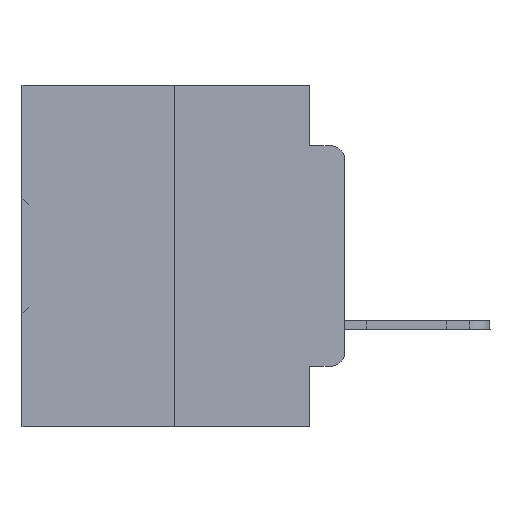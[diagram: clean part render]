
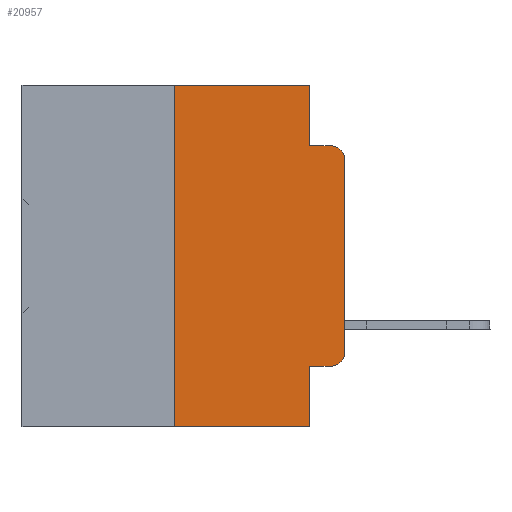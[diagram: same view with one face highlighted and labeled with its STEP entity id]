
A CAD part, left-side view. The second image highlights one B-rep face of the part: STEP entity #20957.
In plain terms, the highlighted planar face has unit normal (-1, 0, 0).
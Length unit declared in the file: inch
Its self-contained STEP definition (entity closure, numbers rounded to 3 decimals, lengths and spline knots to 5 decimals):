
#262 = DIRECTION ( 'NONE',  ( 0., -1., 0. ) ) ;
#642 = EDGE_CURVE ( 'NONE', #31950, #31048, #36042, .T. ) ;
#1874 = DIRECTION ( 'NONE',  ( -1., 0., 0. ) ) ;
#1980 = EDGE_CURVE ( 'NONE', #3647, #34408, #6090, .T. ) ;
#2743 = ORIENTED_EDGE ( 'NONE', *, *, #1980, .F. ) ;
#2965 = ORIENTED_EDGE ( 'NONE', *, *, #6004, .T. ) ;
#3647 = VERTEX_POINT ( 'NONE', #27673 ) ;
#4085 = VECTOR ( 'NONE', #11490, 39.37008 ) ;
#4771 = EDGE_CURVE ( 'NONE', #16785, #33206, #8802, .T. ) ;
#5442 = ORIENTED_EDGE ( 'NONE', *, *, #27793, .F. ) ;
#6004 = EDGE_CURVE ( 'NONE', #22142, #33494, #24230, .T. ) ;
#6090 = LINE ( 'NONE', #29186, #32910 ) ;
#6356 = PLANE ( 'NONE',  #19938 ) ;
#7488 = EDGE_LOOP ( 'NONE', ( #9934, #19368, #13056, #5442, #2743, #19041, #13561, #19748, #2965, #9713 ) ) ;
#7944 = CIRCLE ( 'NONE', #23440, 0.02 ) ;
#8224 = VECTOR ( 'NONE', #30448, 39.37008 ) ;
#8802 = LINE ( 'NONE', #28717, #4085 ) ;
#8894 = DIRECTION ( 'NONE',  ( 0., -1., 0. ) ) ;
#9002 = LINE ( 'NONE', #22781, #23582 ) ;
#9028 = DIRECTION ( 'NONE',  ( -1., 0., 0. ) ) ;
#9069 = VERTEX_POINT ( 'NONE', #16126 ) ;
#9713 = ORIENTED_EDGE ( 'NONE', *, *, #20241, .T. ) ;
#9934 = ORIENTED_EDGE ( 'NONE', *, *, #642, .T. ) ;
#10415 = VERTEX_POINT ( 'NONE', #25073 ) ;
#10775 = EDGE_CURVE ( 'NONE', #16785, #3647, #13095, .T. ) ;
#10931 = CARTESIAN_POINT ( 'NONE',  ( 0., 0.02, -0.4115 ) ) ;
#11490 = DIRECTION ( 'NONE',  ( 0., -1., 0. ) ) ;
#13056 = ORIENTED_EDGE ( 'NONE', *, *, #24681, .F. ) ;
#13095 = LINE ( 'NONE', #13651, #34116 ) ;
#13189 = DIRECTION ( 'NONE',  ( 0., 0., -1. ) ) ;
#13380 = CARTESIAN_POINT ( 'NONE',  ( 0., 0.051, -0.4115 ) ) ;
#13561 = ORIENTED_EDGE ( 'NONE', *, *, #4771, .T. ) ;
#13651 = CARTESIAN_POINT ( 'NONE',  ( 0., 0.25, 0. ) ) ;
#14601 = CARTESIAN_POINT ( 'NONE',  ( 0., 0.02, -0.1085 ) ) ;
#14711 = DIRECTION ( 'NONE',  ( 1., 0., 0. ) ) ;
#15269 = FACE_OUTER_BOUND ( 'NONE', #7488, .T. ) ;
#16126 = CARTESIAN_POINT ( 'NONE',  ( 0., 0.051, -0.0885 ) ) ;
#16474 = DIRECTION ( 'NONE',  ( 0., 0., 1. ) ) ;
#16520 = AXIS2_PLACEMENT_3D ( 'NONE', #14601, #9028, #20409 ) ;
#16656 = CARTESIAN_POINT ( 'NONE',  ( 0., 0.25, -0.5 ) ) ;
#16785 = VERTEX_POINT ( 'NONE', #16656 ) ;
#19041 = ORIENTED_EDGE ( 'NONE', *, *, #10775, .F. ) ;
#19187 = DIRECTION ( 'NONE',  ( 0., -1., 0. ) ) ;
#19368 = ORIENTED_EDGE ( 'NONE', *, *, #29441, .T. ) ;
#19748 = ORIENTED_EDGE ( 'NONE', *, *, #23740, .F. ) ;
#19938 = AXIS2_PLACEMENT_3D ( 'NONE', #20718, #14711, #26094 ) ;
#20034 = LINE ( 'NONE', #28582, #25477 ) ;
#20241 = EDGE_CURVE ( 'NONE', #33494, #31950, #7944, .T. ) ;
#20409 = DIRECTION ( 'NONE',  ( 0., 0., -1. ) ) ;
#20718 = CARTESIAN_POINT ( 'NONE',  ( 0., 0.473, 0. ) ) ;
#20864 = DIRECTION ( 'NONE',  ( 0., 0., -1. ) ) ;
#20957 = ADVANCED_FACE ( 'NONE', ( #15269 ), #6356, .F. ) ;
#21107 = CARTESIAN_POINT ( 'NONE',  ( 0., 0., -0.1085 ) ) ;
#22142 = VERTEX_POINT ( 'NONE', #27848 ) ;
#22545 = CARTESIAN_POINT ( 'NONE',  ( 0., 0.051, -0.5 ) ) ;
#22781 = CARTESIAN_POINT ( 'NONE',  ( 0., 0.051, 0. ) ) ;
#23440 = AXIS2_PLACEMENT_3D ( 'NONE', #27391, #1874, #13189 ) ;
#23582 = VECTOR ( 'NONE', #26139, 39.37008 ) ;
#23740 = EDGE_CURVE ( 'NONE', #22142, #33206, #31070, .T. ) ;
#24230 = LINE ( 'NONE', #13380, #30600 ) ;
#24681 = EDGE_CURVE ( 'NONE', #9069, #10415, #20034, .T. ) ;
#25073 = CARTESIAN_POINT ( 'NONE',  ( 0., 0.02, -0.0885 ) ) ;
#25477 = VECTOR ( 'NONE', #262, 39.37008 ) ;
#26094 = DIRECTION ( 'NONE',  ( 0., 0., -1. ) ) ;
#26139 = DIRECTION ( 'NONE',  ( 0., 0., -1. ) ) ;
#26208 = CARTESIAN_POINT ( 'NONE',  ( 0., 0.051, 0. ) ) ;
#26250 = CARTESIAN_POINT ( 'NONE',  ( 0., 0.051, 0. ) ) ;
#27391 = CARTESIAN_POINT ( 'NONE',  ( 0., 0.02, -0.3915 ) ) ;
#27482 = CARTESIAN_POINT ( 'NONE',  ( 0., 0., 0. ) ) ;
#27673 = CARTESIAN_POINT ( 'NONE',  ( 0., 0.25, 0. ) ) ;
#27793 = EDGE_CURVE ( 'NONE', #34408, #9069, #9002, .T. ) ;
#27848 = CARTESIAN_POINT ( 'NONE',  ( 0., 0.051, -0.4115 ) ) ;
#28582 = CARTESIAN_POINT ( 'NONE',  ( 0., 0.051, -0.0885 ) ) ;
#28717 = CARTESIAN_POINT ( 'NONE',  ( 0., 0.473, -0.5 ) ) ;
#29186 = CARTESIAN_POINT ( 'NONE',  ( 0., 0.473, 0. ) ) ;
#29441 = EDGE_CURVE ( 'NONE', #31048, #10415, #32578, .T. ) ;
#30448 = DIRECTION ( 'NONE',  ( 0., 0., 1. ) ) ;
#30600 = VECTOR ( 'NONE', #19187, 39.37008 ) ;
#30792 = VECTOR ( 'NONE', #20864, 39.37008 ) ;
#31048 = VERTEX_POINT ( 'NONE', #21107 ) ;
#31070 = LINE ( 'NONE', #26250, #30792 ) ;
#31950 = VERTEX_POINT ( 'NONE', #36252 ) ;
#32578 = CIRCLE ( 'NONE', #16520, 0.02 ) ;
#32910 = VECTOR ( 'NONE', #8894, 39.37008 ) ;
#33206 = VERTEX_POINT ( 'NONE', #22545 ) ;
#33494 = VERTEX_POINT ( 'NONE', #10931 ) ;
#34116 = VECTOR ( 'NONE', #16474, 39.37008 ) ;
#34408 = VERTEX_POINT ( 'NONE', #26208 ) ;
#36042 = LINE ( 'NONE', #27482, #8224 ) ;
#36252 = CARTESIAN_POINT ( 'NONE',  ( 0., 0., -0.3915 ) ) ;
